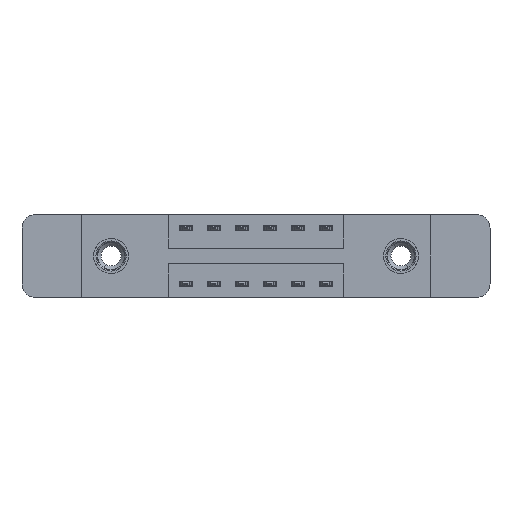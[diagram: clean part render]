
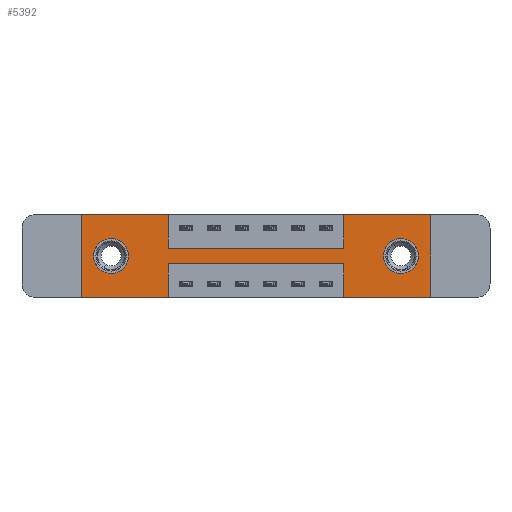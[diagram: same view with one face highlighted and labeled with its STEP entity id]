
A CAD part, front view. The second image highlights one B-rep face of the part: STEP entity #5392.
In plain terms, the highlighted planar face has unit normal (0, -1, 0).
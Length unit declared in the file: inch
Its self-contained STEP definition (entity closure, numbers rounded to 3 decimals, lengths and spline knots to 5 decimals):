
#109 = DIRECTION ( 'NONE',  ( -1., 0., 0. ) ) ;
#179 = CARTESIAN_POINT ( 'NONE',  ( 0.1325, 0., -0.107 ) ) ;
#427 = LINE ( 'NONE', #5471, #11291 ) ;
#452 = CARTESIAN_POINT ( 'NONE',  ( 0.3875, 0., -0.22 ) ) ;
#649 = VERTEX_POINT ( 'NONE', #6244 ) ;
#792 = DIRECTION ( 'NONE',  ( 0., 0., -1. ) ) ;
#912 = LINE ( 'NONE', #4865, #12305 ) ;
#935 = ORIENTED_EDGE ( 'NONE', *, *, #7815, .T. ) ;
#953 = CARTESIAN_POINT ( 'NONE',  ( 1.1725, 0., -0.15 ) ) ;
#957 = DIRECTION ( 'NONE',  ( 0., 0., 1. ) ) ;
#983 = LINE ( 'NONE', #1470, #9472 ) ;
#1080 = CIRCLE ( 'NONE', #9414, 0.078 ) ;
#1081 = EDGE_CURVE ( 'NONE', #4019, #3445, #6317, .T. ) ;
#1087 = EDGE_LOOP ( 'NONE', ( #4850, #6933, #1819, #5816, #12422, #10962, #8309, #9576, #13507, #9104, #7649, #3167 ) ) ;
#1183 = VERTEX_POINT ( 'NONE', #9461 ) ;
#1317 = EDGE_CURVE ( 'NONE', #3445, #7726, #11750, .T. ) ;
#1470 = CARTESIAN_POINT ( 'NONE',  ( 0.3875, 0., -0.37 ) ) ;
#1692 = VECTOR ( 'NONE', #2281, 39.37008 ) ;
#1788 = CARTESIAN_POINT ( 'NONE',  ( 0.3875, 0., -0.15 ) ) ;
#1819 = ORIENTED_EDGE ( 'NONE', *, *, #4813, .F. ) ;
#2123 = VERTEX_POINT ( 'NONE', #6922 ) ;
#2166 = DIRECTION ( 'NONE',  ( 1., 0., 0. ) ) ;
#2254 = VECTOR ( 'NONE', #6484, 39.37008 ) ;
#2281 = DIRECTION ( 'NONE',  ( 1., 0., 0. ) ) ;
#2461 = DIRECTION ( 'NONE',  ( 0., 0., 1. ) ) ;
#2474 = VECTOR ( 'NONE', #3958, 39.37008 ) ;
#2633 = EDGE_CURVE ( 'NONE', #2123, #5456, #4238, .T. ) ;
#2810 = DIRECTION ( 'NONE',  ( 0., 0., -1. ) ) ;
#2893 = EDGE_CURVE ( 'NONE', #1183, #649, #11096, .T. ) ;
#2960 = VERTEX_POINT ( 'NONE', #3881 ) ;
#3022 = PLANE ( 'NONE',  #12557 ) ;
#3167 = ORIENTED_EDGE ( 'NONE', *, *, #3675, .F. ) ;
#3399 = LINE ( 'NONE', #4536, #10967 ) ;
#3445 = VERTEX_POINT ( 'NONE', #6060 ) ;
#3453 = FACE_BOUND ( 'NONE', #7158, .T. ) ;
#3558 = EDGE_CURVE ( 'NONE', #2960, #4882, #427, .T. ) ;
#3655 = DIRECTION ( 'NONE',  ( 0., 0., 1. ) ) ;
#3675 = EDGE_CURVE ( 'NONE', #11328, #9352, #4037, .T. ) ;
#3804 = VERTEX_POINT ( 'NONE', #4509 ) ;
#3881 = CARTESIAN_POINT ( 'NONE',  ( 0.3875, 0., 0. ) ) ;
#3958 = DIRECTION ( 'NONE',  ( 0., 0., -1. ) ) ;
#4019 = VERTEX_POINT ( 'NONE', #953 ) ;
#4037 = LINE ( 'NONE', #10863, #8870 ) ;
#4113 = CARTESIAN_POINT ( 'NONE',  ( 0., 0., -0.37 ) ) ;
#4139 = CARTESIAN_POINT ( 'NONE',  ( 1.56, 0., 0. ) ) ;
#4238 = LINE ( 'NONE', #12089, #10794 ) ;
#4298 = LINE ( 'NONE', #11935, #9822 ) ;
#4509 = CARTESIAN_POINT ( 'NONE',  ( 0.1325, 0., -0.263 ) ) ;
#4536 = CARTESIAN_POINT ( 'NONE',  ( 0., 0., 0. ) ) ;
#4578 = CARTESIAN_POINT ( 'NONE',  ( 0., 0., 0. ) ) ;
#4666 = DIRECTION ( 'NONE',  ( 0., 1., 0. ) ) ;
#4709 = CARTESIAN_POINT ( 'NONE',  ( 0.3875, 0., -0.37 ) ) ;
#4813 = EDGE_CURVE ( 'NONE', #5456, #12574, #5360, .T. ) ;
#4850 = ORIENTED_EDGE ( 'NONE', *, *, #8604, .F. ) ;
#4851 = AXIS2_PLACEMENT_3D ( 'NONE', #11258, #4666, #8865 ) ;
#4865 = CARTESIAN_POINT ( 'NONE',  ( 0.3875, 0., -0.15 ) ) ;
#4882 = VERTEX_POINT ( 'NONE', #1788 ) ;
#5115 = LINE ( 'NONE', #5481, #2254 ) ;
#5360 = LINE ( 'NONE', #10597, #10847 ) ;
#5392 = ADVANCED_FACE ( 'NONE', ( #6950, #3453, #6053 ), #3022, .T. ) ;
#5456 = VERTEX_POINT ( 'NONE', #11047 ) ;
#5471 = CARTESIAN_POINT ( 'NONE',  ( 0.3875, 0., 0. ) ) ;
#5481 = CARTESIAN_POINT ( 'NONE',  ( 0.3875, 0., -0.22 ) ) ;
#5816 = ORIENTED_EDGE ( 'NONE', *, *, #2633, .F. ) ;
#6053 = FACE_OUTER_BOUND ( 'NONE', #1087, .T. ) ;
#6060 = CARTESIAN_POINT ( 'NONE',  ( 1.1725, 0., 0. ) ) ;
#6085 = VERTEX_POINT ( 'NONE', #179 ) ;
#6244 = CARTESIAN_POINT ( 'NONE',  ( 1.4275, 0., -0.107 ) ) ;
#6317 = LINE ( 'NONE', #7162, #12984 ) ;
#6363 = CARTESIAN_POINT ( 'NONE',  ( 0.1325, 0., -0.185 ) ) ;
#6387 = LINE ( 'NONE', #7429, #2474 ) ;
#6484 = DIRECTION ( 'NONE',  ( -1., 0., 0. ) ) ;
#6572 = EDGE_CURVE ( 'NONE', #9352, #11482, #3399, .T. ) ;
#6648 = ORIENTED_EDGE ( 'NONE', *, *, #11787, .T. ) ;
#6666 = CIRCLE ( 'NONE', #10101, 0.078 ) ;
#6922 = CARTESIAN_POINT ( 'NONE',  ( 1.56, 0., -0.37 ) ) ;
#6933 = ORIENTED_EDGE ( 'NONE', *, *, #13893, .F. ) ;
#6950 = FACE_BOUND ( 'NONE', #10911, .T. ) ;
#7154 = CARTESIAN_POINT ( 'NONE',  ( 0., 0., 0. ) ) ;
#7158 = EDGE_LOOP ( 'NONE', ( #6648, #935 ) ) ;
#7162 = CARTESIAN_POINT ( 'NONE',  ( 1.1725, 0., 0. ) ) ;
#7228 = DIRECTION ( 'NONE',  ( 0., 1., 0. ) ) ;
#7429 = CARTESIAN_POINT ( 'NONE',  ( 1.56, 0., 0. ) ) ;
#7649 = ORIENTED_EDGE ( 'NONE', *, *, #6572, .F. ) ;
#7726 = VERTEX_POINT ( 'NONE', #4139 ) ;
#7815 = EDGE_CURVE ( 'NONE', #3804, #6085, #1080, .T. ) ;
#8261 = DIRECTION ( 'NONE',  ( 0., 1., 0. ) ) ;
#8309 = ORIENTED_EDGE ( 'NONE', *, *, #1081, .F. ) ;
#8604 = EDGE_CURVE ( 'NONE', #9196, #11328, #983, .T. ) ;
#8706 = EDGE_CURVE ( 'NONE', #11482, #2960, #4298, .T. ) ;
#8778 = DIRECTION ( 'NONE',  ( 0., 0., -1. ) ) ;
#8865 = DIRECTION ( 'NONE',  ( 0., 0., 1. ) ) ;
#8870 = VECTOR ( 'NONE', #109, 39.37008 ) ;
#9068 = DIRECTION ( 'NONE',  ( 0., 0., -1. ) ) ;
#9104 = ORIENTED_EDGE ( 'NONE', *, *, #8706, .F. ) ;
#9163 = EDGE_CURVE ( 'NONE', #4882, #4019, #912, .T. ) ;
#9196 = VERTEX_POINT ( 'NONE', #452 ) ;
#9352 = VERTEX_POINT ( 'NONE', #13232 ) ;
#9414 = AXIS2_PLACEMENT_3D ( 'NONE', #6363, #13995, #957 ) ;
#9429 = CARTESIAN_POINT ( 'NONE',  ( 1.4275, 0., -0.185 ) ) ;
#9461 = CARTESIAN_POINT ( 'NONE',  ( 1.4275, 0., -0.263 ) ) ;
#9472 = VECTOR ( 'NONE', #9068, 39.37008 ) ;
#9576 = ORIENTED_EDGE ( 'NONE', *, *, #9163, .F. ) ;
#9822 = VECTOR ( 'NONE', #2166, 39.37008 ) ;
#10101 = AXIS2_PLACEMENT_3D ( 'NONE', #9429, #8261, #2810 ) ;
#10353 = CARTESIAN_POINT ( 'NONE',  ( 1.4275, 0., -0.185 ) ) ;
#10360 = DIRECTION ( 'NONE',  ( 1., 0., 0. ) ) ;
#10378 = CARTESIAN_POINT ( 'NONE',  ( 1.1725, 0., -0.22 ) ) ;
#10430 = DIRECTION ( 'NONE',  ( 0., 0., 1. ) ) ;
#10579 = ORIENTED_EDGE ( 'NONE', *, *, #10836, .T. ) ;
#10597 = CARTESIAN_POINT ( 'NONE',  ( 1.1725, 0., -0.37 ) ) ;
#10794 = VECTOR ( 'NONE', #10880, 39.37008 ) ;
#10796 = CIRCLE ( 'NONE', #4851, 0.078 ) ;
#10836 = EDGE_CURVE ( 'NONE', #649, #1183, #6666, .T. ) ;
#10847 = VECTOR ( 'NONE', #2461, 39.37008 ) ;
#10863 = CARTESIAN_POINT ( 'NONE',  ( 0., 0., -0.37 ) ) ;
#10880 = DIRECTION ( 'NONE',  ( -1., 0., 0. ) ) ;
#10885 = AXIS2_PLACEMENT_3D ( 'NONE', #10353, #7228, #792 ) ;
#10911 = EDGE_LOOP ( 'NONE', ( #10579, #13806 ) ) ;
#10962 = ORIENTED_EDGE ( 'NONE', *, *, #1317, .F. ) ;
#10967 = VECTOR ( 'NONE', #3655, 39.37008 ) ;
#11047 = CARTESIAN_POINT ( 'NONE',  ( 1.1725, 0., -0.37 ) ) ;
#11096 = CIRCLE ( 'NONE', #10885, 0.078 ) ;
#11258 = CARTESIAN_POINT ( 'NONE',  ( 0.1325, 0., -0.185 ) ) ;
#11291 = VECTOR ( 'NONE', #8778, 39.37008 ) ;
#11328 = VERTEX_POINT ( 'NONE', #4709 ) ;
#11482 = VERTEX_POINT ( 'NONE', #7154 ) ;
#11750 = LINE ( 'NONE', #4578, #1692 ) ;
#11787 = EDGE_CURVE ( 'NONE', #6085, #3804, #10796, .T. ) ;
#11935 = CARTESIAN_POINT ( 'NONE',  ( 0., 0., 0. ) ) ;
#12089 = CARTESIAN_POINT ( 'NONE',  ( 0., 0., -0.37 ) ) ;
#12305 = VECTOR ( 'NONE', #10360, 39.37008 ) ;
#12422 = ORIENTED_EDGE ( 'NONE', *, *, #12690, .F. ) ;
#12557 = AXIS2_PLACEMENT_3D ( 'NONE', #4113, #12818, #12959 ) ;
#12574 = VERTEX_POINT ( 'NONE', #10378 ) ;
#12690 = EDGE_CURVE ( 'NONE', #7726, #2123, #6387, .T. ) ;
#12818 = DIRECTION ( 'NONE',  ( 0., -1., 0. ) ) ;
#12959 = DIRECTION ( 'NONE',  ( 0., 0., -1. ) ) ;
#12984 = VECTOR ( 'NONE', #10430, 39.37008 ) ;
#13232 = CARTESIAN_POINT ( 'NONE',  ( 0., 0., -0.37 ) ) ;
#13507 = ORIENTED_EDGE ( 'NONE', *, *, #3558, .F. ) ;
#13806 = ORIENTED_EDGE ( 'NONE', *, *, #2893, .T. ) ;
#13893 = EDGE_CURVE ( 'NONE', #12574, #9196, #5115, .T. ) ;
#13995 = DIRECTION ( 'NONE',  ( 0., 1., 0. ) ) ;
